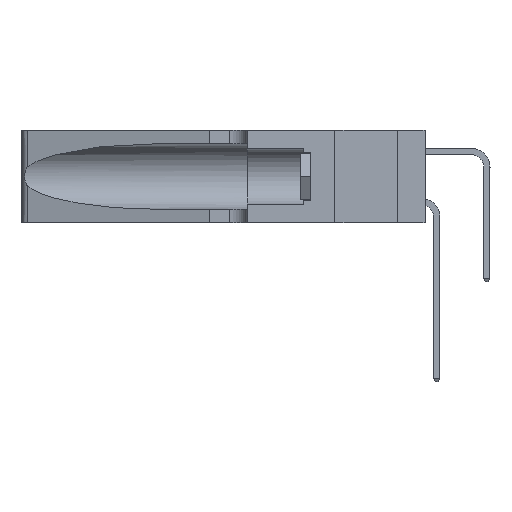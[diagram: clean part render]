
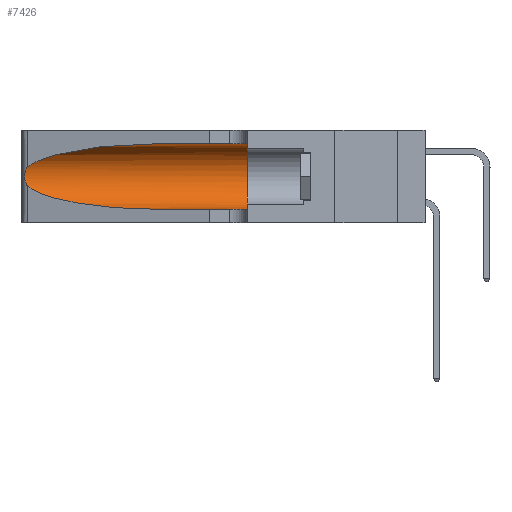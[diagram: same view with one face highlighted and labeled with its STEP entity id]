
A CAD part, left-side view. The second image highlights one B-rep face of the part: STEP entity #7426.
In plain terms, the highlighted cylindrical face has radius 3.308 mm (diameter 6.617 mm), a partial arc.
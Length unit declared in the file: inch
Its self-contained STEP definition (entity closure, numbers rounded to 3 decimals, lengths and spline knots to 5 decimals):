
#345 =( BOUNDED_CURVE ( )  B_SPLINE_CURVE ( 3, ( #40691, #24420, #21026, #4335 ),
 .UNSPECIFIED., .F., .F. ) 
 B_SPLINE_CURVE_WITH_KNOTS ( ( 4, 4 ),
 ( 3.44316, 4.71239 ),
 .UNSPECIFIED. ) 
 CURVE ( )  GEOMETRIC_REPRESENTATION_ITEM ( )  RATIONAL_B_SPLINE_CURVE ( ( 1., 0.87, 0.87, 1. ) ) 
 REPRESENTATION_ITEM ( '' )  );
#1148 = B_SPLINE_CURVE_WITH_KNOTS ( 'NONE', 3,
 ( #41512, #37668, #14358, #7727, #37817, #17713, #21090, #21404, #31242, #9010, #35099, #1625, #28159, #19008 ),
 .UNSPECIFIED., .F., .F.,
 ( 4, 2, 2, 2, 2, 2, 4 ),
 ( 0., 0.00027, 0.00053, 0.00107, 0.0016, 0.00187, 0.00214 ),
 .UNSPECIFIED. ) ;
#1230 = VERTEX_POINT ( 'NONE', #36437 ) ;
#1300 = CARTESIAN_POINT ( 'NONE',  ( 0.1305, 1.61858, 0.185 ) ) ;
#1625 = CARTESIAN_POINT ( 'NONE',  ( 0.25639, 1.23186, 0.15144 ) ) ;
#1864 = DIRECTION ( 'NONE',  ( 0., -1., 0. ) ) ;
#1897 = ORIENTED_EDGE ( 'NONE', *, *, #30798, .T. ) ;
#2101 = DIRECTION ( 'NONE',  ( 0., -1., 0. ) ) ;
#2417 = CARTESIAN_POINT ( 'NONE',  ( 0.1305, 0.72297, 0.31525 ) ) ;
#2603 = EDGE_CURVE ( 'NONE', #39979, #25991, #345, .T. ) ;
#2754 = VERTEX_POINT ( 'NONE', #25736 ) ;
#4335 = CARTESIAN_POINT ( 'NONE',  ( 0.1305, 0.72297, 0.05475 ) ) ;
#5504 = CARTESIAN_POINT ( 'NONE',  ( 0.25487, 1.22718, 0.22369 ) ) ;
#7426 = ADVANCED_FACE ( 'NONE', ( #25472 ), #13346, .F. ) ;
#7727 = CARTESIAN_POINT ( 'NONE',  ( 0.25787, 1.23484, 0.2124 ) ) ;
#7994 = ORIENTED_EDGE ( 'NONE', *, *, #2603, .T. ) ;
#8710 = VECTOR ( 'NONE', #2101, 39.37008 ) ;
#9010 = CARTESIAN_POINT ( 'NONE',  ( 0.25856, 1.23593, 0.16098 ) ) ;
#9680 = ORIENTED_EDGE ( 'NONE', *, *, #36451, .T. ) ;
#9765 = LINE ( 'NONE', #22212, #8710 ) ;
#11947 = DIRECTION ( 'NONE',  ( 0., -1., 0. ) ) ;
#12028 = VECTOR ( 'NONE', #1864, 39.37008 ) ;
#13346 = CYLINDRICAL_SURFACE ( 'NONE', #30089, 0.13025 ) ;
#13378 = DIRECTION ( 'NONE',  ( 0., 0., -1. ) ) ;
#14358 = CARTESIAN_POINT ( 'NONE',  ( 0.25639, 1.23184, 0.21858 ) ) ;
#14460 = CARTESIAN_POINT ( 'NONE',  ( 0.1305, 0.35, 0.185 ) ) ;
#15187 = CARTESIAN_POINT ( 'NONE',  ( 0.1305, 1.61858, 0.05475 ) ) ;
#16524 = ORIENTED_EDGE ( 'NONE', *, *, #33225, .T. ) ;
#16790 = CARTESIAN_POINT ( 'NONE',  ( 0.1305, 0.35, 0.05475 ) ) ;
#17027 = EDGE_CURVE ( 'NONE', #2754, #36010, #33521, .T. ) ;
#17377 = DIRECTION ( 'NONE',  ( 0., 1., 0. ) ) ;
#17713 = CARTESIAN_POINT ( 'NONE',  ( 0.26018, 1.23835, 0.19895 ) ) ;
#18272 = AXIS2_PLACEMENT_3D ( 'NONE', #14460, #17377, #40851 ) ;
#19008 = CARTESIAN_POINT ( 'NONE',  ( 0.25487, 1.22718, 0.14631 ) ) ;
#19938 = ORIENTED_EDGE ( 'NONE', *, *, #17027, .F. ) ;
#21026 = CARTESIAN_POINT ( 'NONE',  ( 0.18966, 0.96281, 0.05475 ) ) ;
#21090 = CARTESIAN_POINT ( 'NONE',  ( 0.26075, 1.23896, 0.19203 ) ) ;
#21404 = CARTESIAN_POINT ( 'NONE',  ( 0.26075, 1.23896, 0.178 ) ) ;
#22212 = CARTESIAN_POINT ( 'NONE',  ( 0.1305, 1.61858, 0.31525 ) ) ;
#24420 = CARTESIAN_POINT ( 'NONE',  ( 0.2373, 1.15595, 0.08982 ) ) ;
#24553 =( BOUNDED_CURVE ( )  B_SPLINE_CURVE ( 3, ( #2417, #39217, #42323, #5504 ),
 .UNSPECIFIED., .F., .F. ) 
 B_SPLINE_CURVE_WITH_KNOTS ( ( 4, 4 ),
 ( 1.5708, 2.84003 ),
 .UNSPECIFIED. ) 
 CURVE ( )  GEOMETRIC_REPRESENTATION_ITEM ( )  RATIONAL_B_SPLINE_CURVE ( ( 1., 0.87, 0.87, 1. ) ) 
 REPRESENTATION_ITEM ( '' )  );
#25472 = FACE_OUTER_BOUND ( 'NONE', #27610, .T. ) ;
#25736 = CARTESIAN_POINT ( 'NONE',  ( 0.1305, 0.35, 0.31525 ) ) ;
#25991 = VERTEX_POINT ( 'NONE', #34151 ) ;
#26922 = VERTEX_POINT ( 'NONE', #32483 ) ;
#27610 = EDGE_LOOP ( 'NONE', ( #9680, #1897, #7994, #16524, #19938, #29919 ) ) ;
#28159 = CARTESIAN_POINT ( 'NONE',  ( 0.25555, 1.22993, 0.14849 ) ) ;
#28521 = EDGE_CURVE ( 'NONE', #1230, #2754, #9765, .T. ) ;
#29919 = ORIENTED_EDGE ( 'NONE', *, *, #28521, .F. ) ;
#30089 = AXIS2_PLACEMENT_3D ( 'NONE', #1300, #11947, #13378 ) ;
#30798 = EDGE_CURVE ( 'NONE', #26922, #39979, #1148, .T. ) ;
#31242 = CARTESIAN_POINT ( 'NONE',  ( 0.26017, 1.23833, 0.17102 ) ) ;
#32483 = CARTESIAN_POINT ( 'NONE',  ( 0.25487, 1.22718, 0.22369 ) ) ;
#33225 = EDGE_CURVE ( 'NONE', #25991, #36010, #37169, .T. ) ;
#33521 = CIRCLE ( 'NONE', #18272, 0.13025 ) ;
#34151 = CARTESIAN_POINT ( 'NONE',  ( 0.1305, 0.72297, 0.05475 ) ) ;
#35099 = CARTESIAN_POINT ( 'NONE',  ( 0.25789, 1.23486, 0.15765 ) ) ;
#36010 = VERTEX_POINT ( 'NONE', #16790 ) ;
#36186 = CARTESIAN_POINT ( 'NONE',  ( 0.25487, 1.22718, 0.14631 ) ) ;
#36437 = CARTESIAN_POINT ( 'NONE',  ( 0.1305, 0.72297, 0.31525 ) ) ;
#36451 = EDGE_CURVE ( 'NONE', #1230, #26922, #24553, .T. ) ;
#37169 = LINE ( 'NONE', #15187, #12028 ) ;
#37668 = CARTESIAN_POINT ( 'NONE',  ( 0.25555, 1.22994, 0.2215 ) ) ;
#37817 = CARTESIAN_POINT ( 'NONE',  ( 0.25854, 1.2359, 0.20912 ) ) ;
#39217 = CARTESIAN_POINT ( 'NONE',  ( 0.18966, 0.96281, 0.31525 ) ) ;
#39979 = VERTEX_POINT ( 'NONE', #36186 ) ;
#40691 = CARTESIAN_POINT ( 'NONE',  ( 0.25487, 1.22718, 0.14631 ) ) ;
#40851 = DIRECTION ( 'NONE',  ( 0., 0., 1. ) ) ;
#41512 = CARTESIAN_POINT ( 'NONE',  ( 0.25487, 1.22718, 0.22369 ) ) ;
#42323 = CARTESIAN_POINT ( 'NONE',  ( 0.2373, 1.15595, 0.28018 ) ) ;
